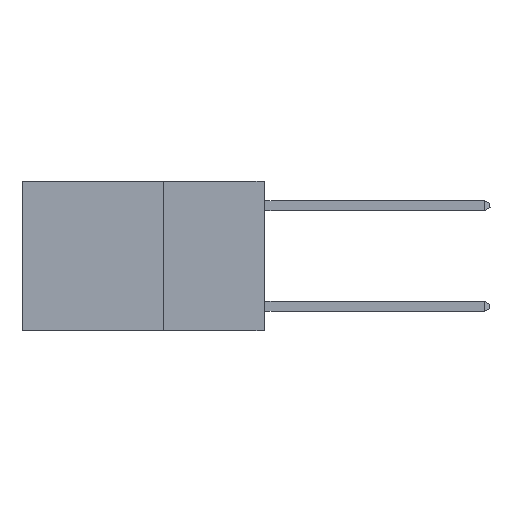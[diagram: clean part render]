
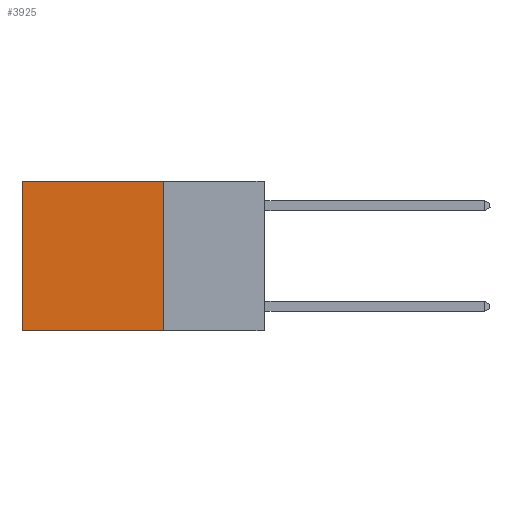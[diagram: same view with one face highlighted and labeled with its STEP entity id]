
A CAD part, left-side view. The second image highlights one B-rep face of the part: STEP entity #3925.
In plain terms, the highlighted planar face has unit normal (-1, 0, 0).
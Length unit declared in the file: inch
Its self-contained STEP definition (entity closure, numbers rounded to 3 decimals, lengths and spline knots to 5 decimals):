
#153 = ORIENTED_EDGE ( 'NONE', *, *, #5286, .T. ) ;
#1400 = EDGE_CURVE ( 'NONE', #1728, #15090, #16452, .T. ) ;
#1728 = VERTEX_POINT ( 'NONE', #26811 ) ;
#1817 = VECTOR ( 'NONE', #14250, 39.37008 ) ;
#2417 = CARTESIAN_POINT ( 'NONE',  ( 0.2625, 0.25, 0. ) ) ;
#2592 = DIRECTION ( 'NONE',  ( 0., 0., -1. ) ) ;
#3045 = DIRECTION ( 'NONE',  ( 0., 0., -1. ) ) ;
#3925 = ADVANCED_FACE ( 'NONE', ( #24852 ), #5962, .F. ) ;
#4354 = AXIS2_PLACEMENT_3D ( 'NONE', #21159, #14931, #7966 ) ;
#4598 = LINE ( 'NONE', #23167, #1817 ) ;
#5072 = ORIENTED_EDGE ( 'NONE', *, *, #1400, .T. ) ;
#5286 = EDGE_CURVE ( 'NONE', #15090, #6658, #13443, .T. ) ;
#5889 = VECTOR ( 'NONE', #2592, 39.37008 ) ;
#5962 = PLANE ( 'NONE',  #4354 ) ;
#6535 = EDGE_CURVE ( 'NONE', #1728, #18786, #14518, .T. ) ;
#6658 = VERTEX_POINT ( 'NONE', #20396 ) ;
#7201 = CARTESIAN_POINT ( 'NONE',  ( 0.2625, 0.25, 0. ) ) ;
#7966 = DIRECTION ( 'NONE',  ( 0., 0., -1. ) ) ;
#8303 = ORIENTED_EDGE ( 'NONE', *, *, #6535, .F. ) ;
#12392 = CARTESIAN_POINT ( 'NONE',  ( 0.2625, 0.25, -0.37 ) ) ;
#12773 = CARTESIAN_POINT ( 'NONE',  ( 0.2625, 0.6, 0. ) ) ;
#12776 = VECTOR ( 'NONE', #3045, 39.37008 ) ;
#13443 = LINE ( 'NONE', #12773, #12776 ) ;
#13662 = DIRECTION ( 'NONE',  ( 0., 1., 0. ) ) ;
#13854 = EDGE_LOOP ( 'NONE', ( #153, #27791, #8303, #5072 ) ) ;
#14250 = DIRECTION ( 'NONE',  ( 0., 1., 0. ) ) ;
#14518 = LINE ( 'NONE', #2417, #5889 ) ;
#14931 = DIRECTION ( 'NONE',  ( 1., 0., 0. ) ) ;
#15090 = VERTEX_POINT ( 'NONE', #25411 ) ;
#15474 = EDGE_CURVE ( 'NONE', #18786, #6658, #4598, .T. ) ;
#16452 = LINE ( 'NONE', #7201, #25017 ) ;
#18786 = VERTEX_POINT ( 'NONE', #12392 ) ;
#20396 = CARTESIAN_POINT ( 'NONE',  ( 0.2625, 0.6, -0.37 ) ) ;
#21159 = CARTESIAN_POINT ( 'NONE',  ( 0.2625, 0.25, 0. ) ) ;
#23167 = CARTESIAN_POINT ( 'NONE',  ( 0.2625, 0.25, -0.37 ) ) ;
#24852 = FACE_OUTER_BOUND ( 'NONE', #13854, .T. ) ;
#25017 = VECTOR ( 'NONE', #13662, 39.37008 ) ;
#25411 = CARTESIAN_POINT ( 'NONE',  ( 0.2625, 0.6, 0. ) ) ;
#26811 = CARTESIAN_POINT ( 'NONE',  ( 0.2625, 0.25, 0. ) ) ;
#27791 = ORIENTED_EDGE ( 'NONE', *, *, #15474, .F. ) ;
